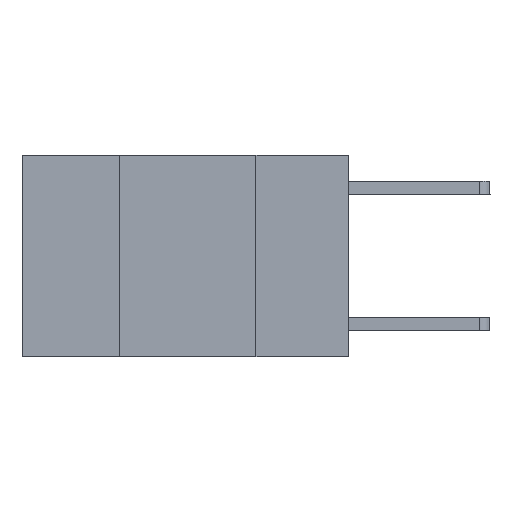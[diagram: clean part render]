
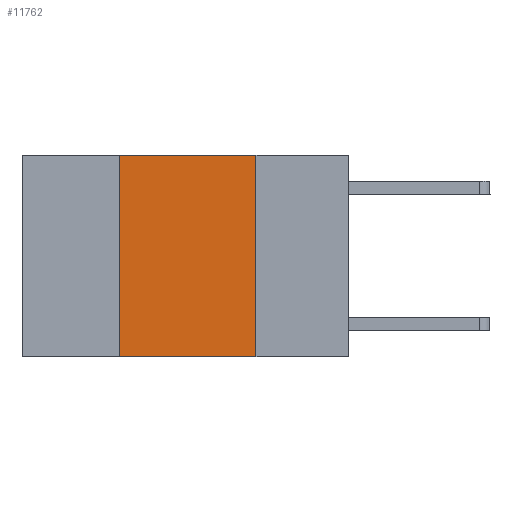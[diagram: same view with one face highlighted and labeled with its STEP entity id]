
A CAD part, left-side view. The second image highlights one B-rep face of the part: STEP entity #11762.
In plain terms, the highlighted planar face has unit normal (-1, 0, 0).
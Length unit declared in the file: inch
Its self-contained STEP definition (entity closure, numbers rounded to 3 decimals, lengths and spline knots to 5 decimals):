
#548 = DIRECTION ( 'NONE',  ( 0., -1., 0. ) ) ;
#1054 = VECTOR ( 'NONE', #548, 39.37008 ) ;
#1868 = CARTESIAN_POINT ( 'NONE',  ( 0., 0.17, 0. ) ) ;
#2166 = LINE ( 'NONE', #5333, #1054 ) ;
#2491 = EDGE_LOOP ( 'NONE', ( #7143, #6651, #4003, #4592 ) ) ;
#2641 = LINE ( 'NONE', #5463, #6090 ) ;
#2854 = LINE ( 'NONE', #9274, #5515 ) ;
#3492 = VERTEX_POINT ( 'NONE', #8185 ) ;
#4003 = ORIENTED_EDGE ( 'NONE', *, *, #9140, .F. ) ;
#4124 = EDGE_CURVE ( 'NONE', #5747, #3492, #2166, .T. ) ;
#4156 = DIRECTION ( 'NONE',  ( 1., 0., 0. ) ) ;
#4592 = ORIENTED_EDGE ( 'NONE', *, *, #4124, .T. ) ;
#4965 = CARTESIAN_POINT ( 'NONE',  ( 0., 0.42, 0. ) ) ;
#5149 = FACE_OUTER_BOUND ( 'NONE', #2491, .T. ) ;
#5166 = AXIS2_PLACEMENT_3D ( 'NONE', #5322, #4156, #7950 ) ;
#5322 = CARTESIAN_POINT ( 'NONE',  ( 0., 0.6, 0. ) ) ;
#5333 = CARTESIAN_POINT ( 'NONE',  ( 0., 0.6, -0.37 ) ) ;
#5463 = CARTESIAN_POINT ( 'NONE',  ( 0., 0.42, 0. ) ) ;
#5515 = VECTOR ( 'NONE', #8491, 39.37008 ) ;
#5747 = VERTEX_POINT ( 'NONE', #7818 ) ;
#5863 = LINE ( 'NONE', #8607, #9451 ) ;
#6090 = VECTOR ( 'NONE', #10679, 39.37008 ) ;
#6178 = EDGE_CURVE ( 'NONE', #7664, #3492, #5863, .T. ) ;
#6651 = ORIENTED_EDGE ( 'NONE', *, *, #9323, .F. ) ;
#7143 = ORIENTED_EDGE ( 'NONE', *, *, #6178, .F. ) ;
#7664 = VERTEX_POINT ( 'NONE', #1868 ) ;
#7818 = CARTESIAN_POINT ( 'NONE',  ( 0., 0.42, -0.37 ) ) ;
#7950 = DIRECTION ( 'NONE',  ( 0., 0., -1. ) ) ;
#8185 = CARTESIAN_POINT ( 'NONE',  ( 0., 0.17, -0.37 ) ) ;
#8491 = DIRECTION ( 'NONE',  ( 0., -1., 0. ) ) ;
#8607 = CARTESIAN_POINT ( 'NONE',  ( 0., 0.17, 0. ) ) ;
#8670 = VERTEX_POINT ( 'NONE', #4965 ) ;
#9140 = EDGE_CURVE ( 'NONE', #5747, #8670, #2641, .T. ) ;
#9274 = CARTESIAN_POINT ( 'NONE',  ( 0., 0.6, 0. ) ) ;
#9323 = EDGE_CURVE ( 'NONE', #8670, #7664, #2854, .T. ) ;
#9451 = VECTOR ( 'NONE', #10508, 39.37008 ) ;
#10508 = DIRECTION ( 'NONE',  ( 0., 0., -1. ) ) ;
#10650 = PLANE ( 'NONE',  #5166 ) ;
#10679 = DIRECTION ( 'NONE',  ( 0., 0., 1. ) ) ;
#11762 = ADVANCED_FACE ( 'NONE', ( #5149 ), #10650, .F. ) ;
